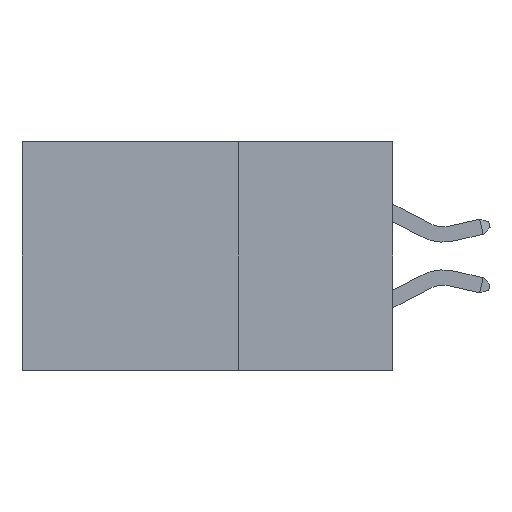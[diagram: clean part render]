
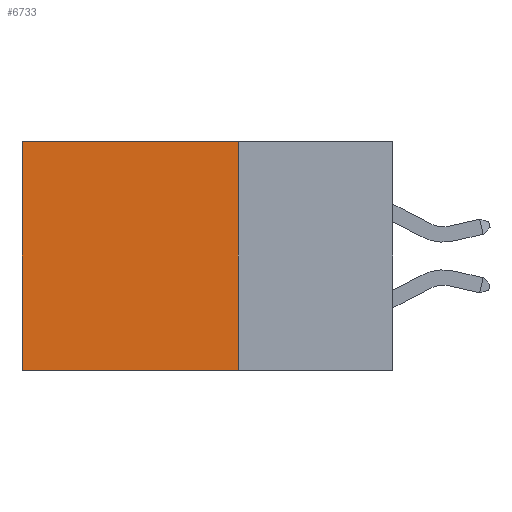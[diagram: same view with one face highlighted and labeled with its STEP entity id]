
A CAD part, left-side view. The second image highlights one B-rep face of the part: STEP entity #6733.
In plain terms, the highlighted planar face has unit normal (-1, 0, 0).
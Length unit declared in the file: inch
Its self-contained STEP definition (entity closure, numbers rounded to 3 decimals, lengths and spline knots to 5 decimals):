
#131 = CARTESIAN_POINT ( 'NONE',  ( 0.2875, 0.25, -0.37 ) ) ;
#247 = DIRECTION ( 'NONE',  ( 0., 1., 0. ) ) ;
#866 = VERTEX_POINT ( 'NONE', #12019 ) ;
#1410 = CARTESIAN_POINT ( 'NONE',  ( 0.2875, 0.6, -0.37 ) ) ;
#1747 = EDGE_CURVE ( 'NONE', #866, #11855, #4991, .T. ) ;
#2351 = DIRECTION ( 'NONE',  ( 1., 0., 0. ) ) ;
#3048 = AXIS2_PLACEMENT_3D ( 'NONE', #14764, #2351, #11158 ) ;
#3311 = VECTOR ( 'NONE', #13424, 39.37008 ) ;
#4035 = DIRECTION ( 'NONE',  ( 0., 0., -1. ) ) ;
#4835 = LINE ( 'NONE', #6496, #14300 ) ;
#4991 = LINE ( 'NONE', #131, #14814 ) ;
#5743 = VERTEX_POINT ( 'NONE', #9049 ) ;
#5999 = ORIENTED_EDGE ( 'NONE', *, *, #10947, .F. ) ;
#6442 = ORIENTED_EDGE ( 'NONE', *, *, #15318, .T. ) ;
#6496 = CARTESIAN_POINT ( 'NONE',  ( 0.2875, 0.6, 0. ) ) ;
#6660 = LINE ( 'NONE', #12181, #3311 ) ;
#6733 = ADVANCED_FACE ( 'NONE', ( #15310 ), #9933, .F. ) ;
#7085 = CARTESIAN_POINT ( 'NONE',  ( 0.2875, 0.25, 0. ) ) ;
#7992 = VERTEX_POINT ( 'NONE', #12158 ) ;
#9049 = CARTESIAN_POINT ( 'NONE',  ( 0.2875, 0.25, 0. ) ) ;
#9933 = PLANE ( 'NONE',  #3048 ) ;
#10656 = VECTOR ( 'NONE', #15651, 39.37008 ) ;
#10947 = EDGE_CURVE ( 'NONE', #5743, #866, #6660, .T. ) ;
#11030 = LINE ( 'NONE', #7085, #10656 ) ;
#11158 = DIRECTION ( 'NONE',  ( 0., 0., -1. ) ) ;
#11855 = VERTEX_POINT ( 'NONE', #1410 ) ;
#12019 = CARTESIAN_POINT ( 'NONE',  ( 0.2875, 0.25, -0.37 ) ) ;
#12158 = CARTESIAN_POINT ( 'NONE',  ( 0.2875, 0.6, 0. ) ) ;
#12181 = CARTESIAN_POINT ( 'NONE',  ( 0.2875, 0.25, 0. ) ) ;
#13424 = DIRECTION ( 'NONE',  ( 0., 0., -1. ) ) ;
#13704 = EDGE_CURVE ( 'NONE', #5743, #7992, #11030, .T. ) ;
#14300 = VECTOR ( 'NONE', #4035, 39.37008 ) ;
#14764 = CARTESIAN_POINT ( 'NONE',  ( 0.2875, 0.25, 0. ) ) ;
#14814 = VECTOR ( 'NONE', #247, 39.37008 ) ;
#14913 = EDGE_LOOP ( 'NONE', ( #6442, #15811, #5999, #15476 ) ) ;
#15310 = FACE_OUTER_BOUND ( 'NONE', #14913, .T. ) ;
#15318 = EDGE_CURVE ( 'NONE', #7992, #11855, #4835, .T. ) ;
#15476 = ORIENTED_EDGE ( 'NONE', *, *, #13704, .T. ) ;
#15651 = DIRECTION ( 'NONE',  ( 0., 1., 0. ) ) ;
#15811 = ORIENTED_EDGE ( 'NONE', *, *, #1747, .F. ) ;
